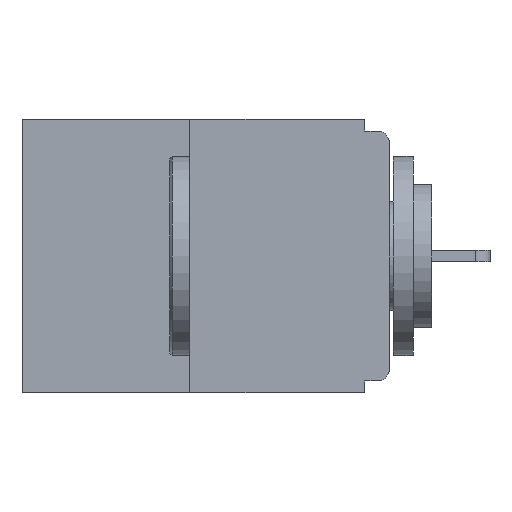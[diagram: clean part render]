
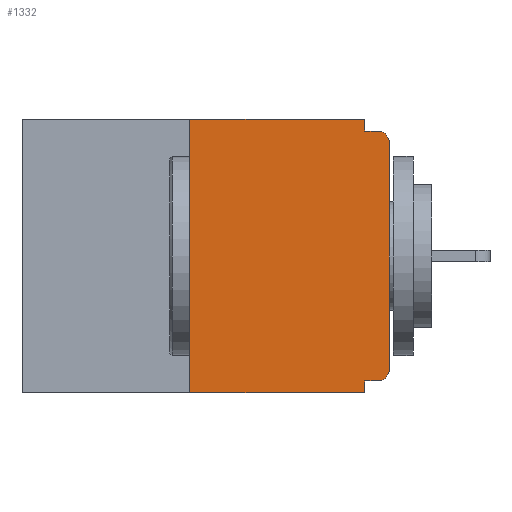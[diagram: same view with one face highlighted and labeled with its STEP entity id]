
A CAD part, left-side view. The second image highlights one B-rep face of the part: STEP entity #1332.
In plain terms, the highlighted planar face has unit normal (-1, 0, 0).
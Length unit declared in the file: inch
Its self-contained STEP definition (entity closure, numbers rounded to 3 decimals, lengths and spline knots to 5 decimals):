
#289 = CARTESIAN_POINT ( 'NONE',  ( 0., 0., -0.015 ) ) ;
#318 = AXIS2_PLACEMENT_3D ( 'NONE', #3685, #15692, #2120 ) ;
#331 = DIRECTION ( 'NONE',  ( 0., 0., 1. ) ) ;
#429 = EDGE_CURVE ( 'NONE', #7258, #12408, #7174, .T. ) ;
#435 = CARTESIAN_POINT ( 'NONE',  ( 0., 0.015, -0.313 ) ) ;
#679 = PLANE ( 'NONE',  #318 ) ;
#684 = VERTEX_POINT ( 'NONE', #10621 ) ;
#819 = LINE ( 'NONE', #17032, #5967 ) ;
#1216 = ORIENTED_EDGE ( 'NONE', *, *, #2113, .T. ) ;
#1332 = ADVANCED_FACE ( 'NONE', ( #12266 ), #679, .F. ) ;
#1339 = VERTEX_POINT ( 'NONE', #11106 ) ;
#1496 = VERTEX_POINT ( 'NONE', #16537 ) ;
#1669 = DIRECTION ( 'NONE',  ( -1., 0., 0. ) ) ;
#2032 = CARTESIAN_POINT ( 'NONE',  ( 0., 0.031, 0. ) ) ;
#2113 = EDGE_CURVE ( 'NONE', #2855, #1496, #9996, .T. ) ;
#2120 = DIRECTION ( 'NONE',  ( 0., 0., -1. ) ) ;
#2440 = LINE ( 'NONE', #5226, #14631 ) ;
#2855 = VERTEX_POINT ( 'NONE', #16204 ) ;
#3326 = VERTEX_POINT ( 'NONE', #16099 ) ;
#3685 = CARTESIAN_POINT ( 'NONE',  ( 0., 0.46, 0. ) ) ;
#3711 = VECTOR ( 'NONE', #18918, 39.37008 ) ;
#4063 = VECTOR ( 'NONE', #19264, 39.37008 ) ;
#4857 = EDGE_CURVE ( 'NONE', #3326, #1496, #15399, .T. ) ;
#5226 = CARTESIAN_POINT ( 'NONE',  ( 0., 0.46, 0. ) ) ;
#5510 = LINE ( 'NONE', #15203, #14627 ) ;
#5886 = CARTESIAN_POINT ( 'NONE',  ( 0., 0.25, 0. ) ) ;
#5967 = VECTOR ( 'NONE', #14289, 39.37008 ) ;
#5998 = ORIENTED_EDGE ( 'NONE', *, *, #13628, .F. ) ;
#6393 = DIRECTION ( 'NONE',  ( 0., 0., -1. ) ) ;
#6787 = ORIENTED_EDGE ( 'NONE', *, *, #9199, .F. ) ;
#6898 = DIRECTION ( 'NONE',  ( 0., -1., 0. ) ) ;
#7174 = CIRCLE ( 'NONE', #14698, 0.015 ) ;
#7258 = VERTEX_POINT ( 'NONE', #10365 ) ;
#7575 = CARTESIAN_POINT ( 'NONE',  ( 0., 0., -0.313 ) ) ;
#7916 = DIRECTION ( 'NONE',  ( 0., -1., 0. ) ) ;
#8033 = LINE ( 'NONE', #5886, #4063 ) ;
#8220 = VERTEX_POINT ( 'NONE', #10986 ) ;
#8299 = CARTESIAN_POINT ( 'NONE',  ( 0., 0.031, -0.343 ) ) ;
#8884 = EDGE_LOOP ( 'NONE', ( #6787, #11607, #1216, #10596, #18123, #18221, #16062, #14260, #13317, #5998 ) ) ;
#9177 = CARTESIAN_POINT ( 'NONE',  ( 0., 0.015, -0.03 ) ) ;
#9199 = EDGE_CURVE ( 'NONE', #15153, #8220, #2440, .T. ) ;
#9249 = EDGE_CURVE ( 'NONE', #7258, #3326, #819, .T. ) ;
#9451 = VECTOR ( 'NONE', #6393, 39.37008 ) ;
#9732 = CARTESIAN_POINT ( 'NONE',  ( 0., 0.46, -0.343 ) ) ;
#9996 = LINE ( 'NONE', #9732, #10240 ) ;
#10075 = LINE ( 'NONE', #289, #16874 ) ;
#10240 = VECTOR ( 'NONE', #6898, 39.37008 ) ;
#10365 = CARTESIAN_POINT ( 'NONE',  ( 0., 0.015, -0.328 ) ) ;
#10596 = ORIENTED_EDGE ( 'NONE', *, *, #4857, .F. ) ;
#10621 = CARTESIAN_POINT ( 'NONE',  ( 0., 0.031, -0.015 ) ) ;
#10755 = VERTEX_POINT ( 'NONE', #18380 ) ;
#10859 = DIRECTION ( 'NONE',  ( 0., 0., -1. ) ) ;
#10986 = CARTESIAN_POINT ( 'NONE',  ( 0., 0.031, 0. ) ) ;
#11083 = DIRECTION ( 'NONE',  ( 0., -1., 0. ) ) ;
#11106 = CARTESIAN_POINT ( 'NONE',  ( 0., 0.015, -0.015 ) ) ;
#11607 = ORIENTED_EDGE ( 'NONE', *, *, #15659, .F. ) ;
#12095 = DIRECTION ( 'NONE',  ( 0., 0., -1. ) ) ;
#12266 = FACE_OUTER_BOUND ( 'NONE', #8884, .T. ) ;
#12408 = VERTEX_POINT ( 'NONE', #7575 ) ;
#12432 = EDGE_CURVE ( 'NONE', #12408, #10755, #5510, .T. ) ;
#12967 = EDGE_CURVE ( 'NONE', #10755, #1339, #13205, .T. ) ;
#13205 = CIRCLE ( 'NONE', #18667, 0.015 ) ;
#13317 = ORIENTED_EDGE ( 'NONE', *, *, #19322, .F. ) ;
#13628 = EDGE_CURVE ( 'NONE', #8220, #684, #15490, .T. ) ;
#14260 = ORIENTED_EDGE ( 'NONE', *, *, #12967, .T. ) ;
#14289 = DIRECTION ( 'NONE',  ( 0., 1., 0. ) ) ;
#14474 = CARTESIAN_POINT ( 'NONE',  ( 0., 0.25, 0. ) ) ;
#14627 = VECTOR ( 'NONE', #331, 39.37008 ) ;
#14631 = VECTOR ( 'NONE', #11083, 39.37008 ) ;
#14698 = AXIS2_PLACEMENT_3D ( 'NONE', #435, #15511, #10859 ) ;
#15153 = VERTEX_POINT ( 'NONE', #14474 ) ;
#15203 = CARTESIAN_POINT ( 'NONE',  ( 0., 0., 0. ) ) ;
#15399 = LINE ( 'NONE', #8299, #3711 ) ;
#15490 = LINE ( 'NONE', #2032, #9451 ) ;
#15511 = DIRECTION ( 'NONE',  ( -1., 0., 0. ) ) ;
#15659 = EDGE_CURVE ( 'NONE', #2855, #15153, #8033, .T. ) ;
#15692 = DIRECTION ( 'NONE',  ( 1., 0., 0. ) ) ;
#16062 = ORIENTED_EDGE ( 'NONE', *, *, #12432, .T. ) ;
#16099 = CARTESIAN_POINT ( 'NONE',  ( 0., 0.031, -0.328 ) ) ;
#16204 = CARTESIAN_POINT ( 'NONE',  ( 0., 0.25, -0.343 ) ) ;
#16537 = CARTESIAN_POINT ( 'NONE',  ( 0., 0.031, -0.343 ) ) ;
#16874 = VECTOR ( 'NONE', #7916, 39.37008 ) ;
#17032 = CARTESIAN_POINT ( 'NONE',  ( 0., 0., -0.328 ) ) ;
#18123 = ORIENTED_EDGE ( 'NONE', *, *, #9249, .F. ) ;
#18221 = ORIENTED_EDGE ( 'NONE', *, *, #429, .T. ) ;
#18380 = CARTESIAN_POINT ( 'NONE',  ( 0., 0., -0.03 ) ) ;
#18667 = AXIS2_PLACEMENT_3D ( 'NONE', #9177, #1669, #12095 ) ;
#18918 = DIRECTION ( 'NONE',  ( 0., 0., -1. ) ) ;
#19264 = DIRECTION ( 'NONE',  ( 0., 0., 1. ) ) ;
#19322 = EDGE_CURVE ( 'NONE', #684, #1339, #10075, .T. ) ;
